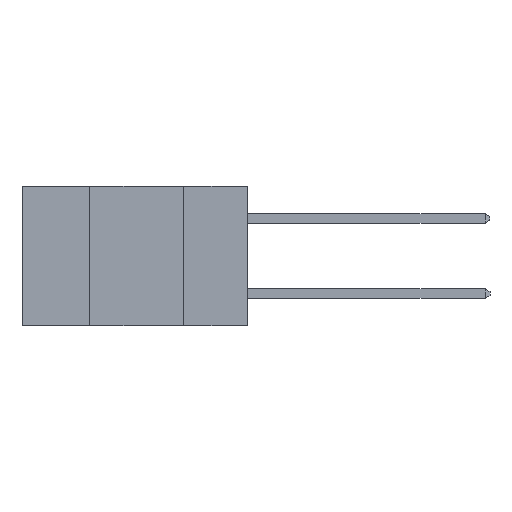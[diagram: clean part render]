
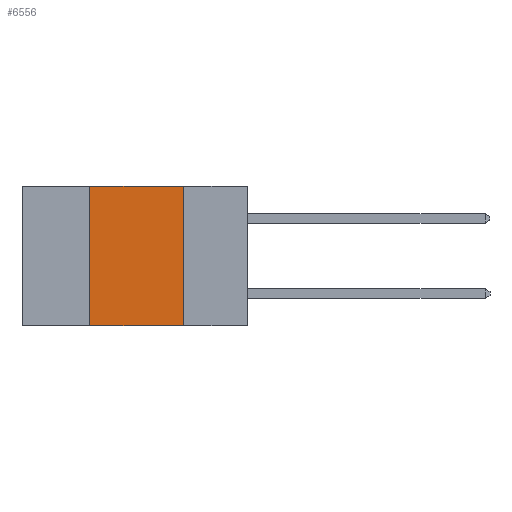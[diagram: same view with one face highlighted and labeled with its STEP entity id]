
A CAD part, left-side view. The second image highlights one B-rep face of the part: STEP entity #6556.
In plain terms, the highlighted planar face has unit normal (-1, 0, 0).
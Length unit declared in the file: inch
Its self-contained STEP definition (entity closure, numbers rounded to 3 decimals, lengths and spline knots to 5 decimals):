
#570 = LINE ( 'NONE', #2427, #2671 ) ;
#795 = VECTOR ( 'NONE', #7007, 39.37008 ) ;
#1134 = VERTEX_POINT ( 'NONE', #7109 ) ;
#1141 = EDGE_CURVE ( 'NONE', #10734, #2535, #3444, .T. ) ;
#1151 = CARTESIAN_POINT ( 'NONE',  ( 0., 0.17, 0. ) ) ;
#2006 = DIRECTION ( 'NONE',  ( 0., 0., -1. ) ) ;
#2008 = DIRECTION ( 'NONE',  ( 1., 0., 0. ) ) ;
#2031 = CARTESIAN_POINT ( 'NONE',  ( 0., 0.6, 0. ) ) ;
#2074 = PLANE ( 'NONE',  #4292 ) ;
#2400 = ORIENTED_EDGE ( 'NONE', *, *, #9706, .T. ) ;
#2427 = CARTESIAN_POINT ( 'NONE',  ( 0., 0.42, -0.37 ) ) ;
#2535 = VERTEX_POINT ( 'NONE', #1151 ) ;
#2671 = VECTOR ( 'NONE', #4163, 39.37008 ) ;
#3333 = FACE_OUTER_BOUND ( 'NONE', #8079, .T. ) ;
#3444 = LINE ( 'NONE', #7080, #795 ) ;
#3461 = VECTOR ( 'NONE', #3958, 39.37008 ) ;
#3656 = DIRECTION ( 'NONE',  ( 0., -1., 0. ) ) ;
#3730 = ORIENTED_EDGE ( 'NONE', *, *, #1141, .F. ) ;
#3958 = DIRECTION ( 'NONE',  ( 0., 0., -1. ) ) ;
#4163 = DIRECTION ( 'NONE',  ( 0., 0., 1. ) ) ;
#4170 = CARTESIAN_POINT ( 'NONE',  ( 0., 0.17, -0.37 ) ) ;
#4292 = AXIS2_PLACEMENT_3D ( 'NONE', #2031, #2008, #2006 ) ;
#4428 = LINE ( 'NONE', #5361, #10518 ) ;
#5361 = CARTESIAN_POINT ( 'NONE',  ( 0., 0.6, -0.37 ) ) ;
#5497 = ORIENTED_EDGE ( 'NONE', *, *, #6236, .F. ) ;
#6236 = EDGE_CURVE ( 'NONE', #2535, #7257, #9927, .T. ) ;
#6276 = CARTESIAN_POINT ( 'NONE',  ( 0., 0.17, -0.37 ) ) ;
#6441 = ORIENTED_EDGE ( 'NONE', *, *, #10199, .F. ) ;
#6556 = ADVANCED_FACE ( 'NONE', ( #3333 ), #2074, .F. ) ;
#7007 = DIRECTION ( 'NONE',  ( 0., -1., 0. ) ) ;
#7080 = CARTESIAN_POINT ( 'NONE',  ( 0., 0.6, 0. ) ) ;
#7109 = CARTESIAN_POINT ( 'NONE',  ( 0., 0.42, -0.37 ) ) ;
#7257 = VERTEX_POINT ( 'NONE', #6276 ) ;
#8079 = EDGE_LOOP ( 'NONE', ( #5497, #3730, #6441, #2400 ) ) ;
#9706 = EDGE_CURVE ( 'NONE', #1134, #7257, #4428, .T. ) ;
#9927 = LINE ( 'NONE', #4170, #3461 ) ;
#10199 = EDGE_CURVE ( 'NONE', #1134, #10734, #570, .T. ) ;
#10518 = VECTOR ( 'NONE', #3656, 39.37008 ) ;
#10717 = CARTESIAN_POINT ( 'NONE',  ( 0., 0.42, 0. ) ) ;
#10734 = VERTEX_POINT ( 'NONE', #10717 ) ;
